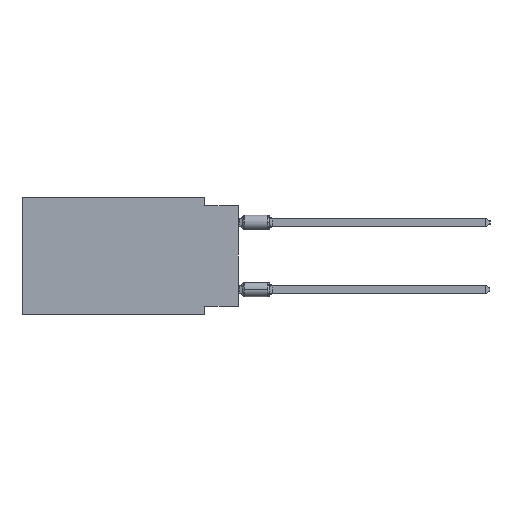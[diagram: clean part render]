
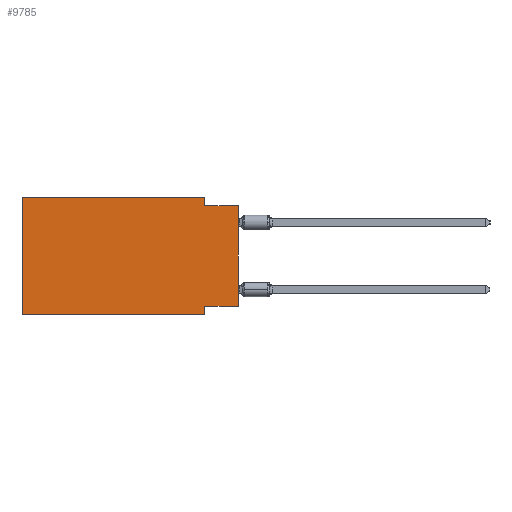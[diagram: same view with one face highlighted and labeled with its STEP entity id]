
A CAD part, left-side view. The second image highlights one B-rep face of the part: STEP entity #9785.
In plain terms, the highlighted planar face has unit normal (-1, 0, 0).
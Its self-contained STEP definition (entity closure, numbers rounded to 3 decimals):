
#24 = CARTESIAN_POINT ( 'NONE',  ( 0., 2.54, -8.89 ) ) ;
#31 = VERTEX_POINT ( 'NONE', #20822 ) ;
#34 = EDGE_CURVE ( 'NONE', #4804, #4177, #17490, .T. ) ;
#76 = VECTOR ( 'NONE', #14050, 1000. ) ;
#449 = EDGE_CURVE ( 'NONE', #4177, #20044, #17972, .T. ) ;
#478 = VECTOR ( 'NONE', #2393, 1000. ) ;
#615 = DIRECTION ( 'NONE',  ( 1., 0., 0. ) ) ;
#1908 = CARTESIAN_POINT ( 'NONE',  ( 0., 16.383, 0. ) ) ;
#2067 = ORIENTED_EDGE ( 'NONE', *, *, #20318, .F. ) ;
#2393 = DIRECTION ( 'NONE',  ( 0., 0., -1. ) ) ;
#2501 = CARTESIAN_POINT ( 'NONE',  ( 0., 16.383, 0. ) ) ;
#2720 = ORIENTED_EDGE ( 'NONE', *, *, #10936, .F. ) ;
#2778 = DIRECTION ( 'NONE',  ( 0., 1., 0. ) ) ;
#2958 = CARTESIAN_POINT ( 'NONE',  ( 0., 2.54, -8.89 ) ) ;
#3103 = ORIENTED_EDGE ( 'NONE', *, *, #21194, .T. ) ;
#3783 = DIRECTION ( 'NONE',  ( 0., -1., 0. ) ) ;
#3939 = VECTOR ( 'NONE', #18490, 1000. ) ;
#4110 = LINE ( 'NONE', #2501, #3939 ) ;
#4177 = VERTEX_POINT ( 'NONE', #7487 ) ;
#4468 = CARTESIAN_POINT ( 'NONE',  ( 0., 2.54, 0. ) ) ;
#4532 = EDGE_LOOP ( 'NONE', ( #3103, #12701, #2067, #2720, #6159, #10975, #12853, #14865 ) ) ;
#4804 = VERTEX_POINT ( 'NONE', #19694 ) ;
#5774 = LINE ( 'NONE', #15875, #76 ) ;
#6159 = ORIENTED_EDGE ( 'NONE', *, *, #17994, .F. ) ;
#6321 = VERTEX_POINT ( 'NONE', #19360 ) ;
#7251 = PLANE ( 'NONE',  #15484 ) ;
#7487 = CARTESIAN_POINT ( 'NONE',  ( 0., 2.54, -8.255 ) ) ;
#8505 = LINE ( 'NONE', #13674, #478 ) ;
#9530 = CARTESIAN_POINT ( 'NONE',  ( 0., 0., -8.255 ) ) ;
#9785 = ADVANCED_FACE ( 'NONE', ( #10589 ), #7251, .F. ) ;
#10589 = FACE_OUTER_BOUND ( 'NONE', #4532, .T. ) ;
#10642 = LINE ( 'NONE', #18488, #12845 ) ;
#10936 = EDGE_CURVE ( 'NONE', #19734, #15999, #13616, .T. ) ;
#10975 = ORIENTED_EDGE ( 'NONE', *, *, #20853, .T. ) ;
#11050 = DIRECTION ( 'NONE',  ( 0., -1., 0. ) ) ;
#12210 = CARTESIAN_POINT ( 'NONE',  ( 0., 16.383, 0. ) ) ;
#12701 = ORIENTED_EDGE ( 'NONE', *, *, #16684, .F. ) ;
#12845 = VECTOR ( 'NONE', #3783, 1000. ) ;
#12853 = ORIENTED_EDGE ( 'NONE', *, *, #449, .F. ) ;
#13385 = DIRECTION ( 'NONE',  ( 0., -1., 0. ) ) ;
#13616 = LINE ( 'NONE', #1908, #16178 ) ;
#13674 = CARTESIAN_POINT ( 'NONE',  ( 0., 2.54, 0. ) ) ;
#14050 = DIRECTION ( 'NONE',  ( 0., 0., 1. ) ) ;
#14150 = VECTOR ( 'NONE', #17761, 1000. ) ;
#14830 = CARTESIAN_POINT ( 'NONE',  ( 0., 2.54, -0.635 ) ) ;
#14865 = ORIENTED_EDGE ( 'NONE', *, *, #34, .F. ) ;
#15010 = CARTESIAN_POINT ( 'NONE',  ( 0., 16.383, 0. ) ) ;
#15484 = AXIS2_PLACEMENT_3D ( 'NONE', #12210, #615, #20239 ) ;
#15875 = CARTESIAN_POINT ( 'NONE',  ( 0., 0., 0. ) ) ;
#15999 = VERTEX_POINT ( 'NONE', #4468 ) ;
#16178 = VECTOR ( 'NONE', #13385, 1000. ) ;
#16684 = EDGE_CURVE ( 'NONE', #17027, #31, #10642, .T. ) ;
#17027 = VERTEX_POINT ( 'NONE', #14830 ) ;
#17189 = LINE ( 'NONE', #20834, #20667 ) ;
#17490 = LINE ( 'NONE', #9530, #21030 ) ;
#17761 = DIRECTION ( 'NONE',  ( 0., 0., -1. ) ) ;
#17972 = LINE ( 'NONE', #24, #14150 ) ;
#17994 = EDGE_CURVE ( 'NONE', #6321, #19734, #4110, .T. ) ;
#18488 = CARTESIAN_POINT ( 'NONE',  ( 0., 0., -0.635 ) ) ;
#18490 = DIRECTION ( 'NONE',  ( 0., 0., 1. ) ) ;
#19360 = CARTESIAN_POINT ( 'NONE',  ( 0., 16.383, -8.89 ) ) ;
#19694 = CARTESIAN_POINT ( 'NONE',  ( 0., 0., -8.255 ) ) ;
#19734 = VERTEX_POINT ( 'NONE', #15010 ) ;
#20044 = VERTEX_POINT ( 'NONE', #2958 ) ;
#20239 = DIRECTION ( 'NONE',  ( 0., 0., -1. ) ) ;
#20318 = EDGE_CURVE ( 'NONE', #15999, #17027, #8505, .T. ) ;
#20667 = VECTOR ( 'NONE', #11050, 1000. ) ;
#20822 = CARTESIAN_POINT ( 'NONE',  ( 0., 0., -0.635 ) ) ;
#20834 = CARTESIAN_POINT ( 'NONE',  ( 0., 16.383, -8.89 ) ) ;
#20853 = EDGE_CURVE ( 'NONE', #6321, #20044, #17189, .T. ) ;
#21030 = VECTOR ( 'NONE', #2778, 1000. ) ;
#21194 = EDGE_CURVE ( 'NONE', #4804, #31, #5774, .T. ) ;
